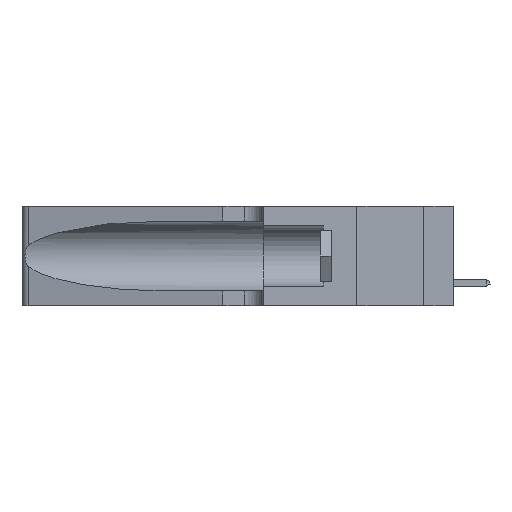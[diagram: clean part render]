
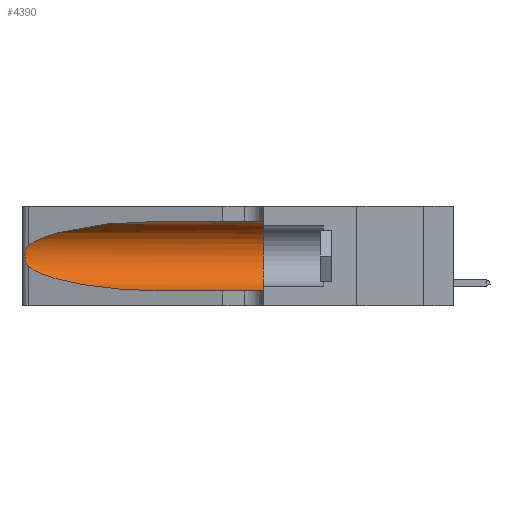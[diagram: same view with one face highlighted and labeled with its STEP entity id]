
A CAD part, left-side view. The second image highlights one B-rep face of the part: STEP entity #4390.
In plain terms, the highlighted cylindrical face has radius 3.308 mm (diameter 6.617 mm), a partial arc.
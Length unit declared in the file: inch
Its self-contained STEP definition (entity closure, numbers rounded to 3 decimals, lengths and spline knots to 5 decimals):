
#173 = CARTESIAN_POINT ( 'NONE',  ( 0.25487, 1.22718, 0.14631 ) ) ;
#246 = CARTESIAN_POINT ( 'NONE',  ( 0.26075, 1.23896, 0.178 ) ) ;
#338 = VERTEX_POINT ( 'NONE', #14343 ) ;
#577 = DIRECTION ( 'NONE',  ( 0., 0., 1. ) ) ;
#1189 = LINE ( 'NONE', #12483, #6958 ) ;
#2213 = CARTESIAN_POINT ( 'NONE',  ( 0.25487, 1.22718, 0.22369 ) ) ;
#2316 = AXIS2_PLACEMENT_3D ( 'NONE', #17102, #3715, #577 ) ;
#2671 = B_SPLINE_CURVE_WITH_KNOTS ( 'NONE', 3,
 ( #15286, #18796, #13555, #13475, #18503, #7005, #17047, #246, #20250, #18652, #7074, #10379, #8681, #8752 ),
 .UNSPECIFIED., .F., .F.,
 ( 4, 2, 2, 2, 2, 2, 4 ),
 ( 0., 0.00027, 0.00053, 0.00107, 0.0016, 0.00187, 0.00214 ),
 .UNSPECIFIED. ) ;
#3072 = CARTESIAN_POINT ( 'NONE',  ( 0.2373, 1.15595, 0.28018 ) ) ;
#3584 = CIRCLE ( 'NONE', #2316, 0.13025 ) ;
#3715 = DIRECTION ( 'NONE',  ( 0., 1., 0. ) ) ;
#4390 = ADVANCED_FACE ( 'NONE', ( #12271 ), #21081, .F. ) ;
#4749 = EDGE_CURVE ( 'NONE', #10232, #21205, #10947, .T. ) ;
#4982 = CARTESIAN_POINT ( 'NONE',  ( 0.1305, 0.35, 0.05475 ) ) ;
#5473 = VERTEX_POINT ( 'NONE', #2213 ) ;
#6452 = ORIENTED_EDGE ( 'NONE', *, *, #4749, .T. ) ;
#6772 = CARTESIAN_POINT ( 'NONE',  ( 0.1305, 1.61858, 0.185 ) ) ;
#6958 = VECTOR ( 'NONE', #9335, 39.37008 ) ;
#6992 = DIRECTION ( 'NONE',  ( 0., 0., -1. ) ) ;
#7005 = CARTESIAN_POINT ( 'NONE',  ( 0.26018, 1.23835, 0.19895 ) ) ;
#7065 = DIRECTION ( 'NONE',  ( 0., -1., 0. ) ) ;
#7074 = CARTESIAN_POINT ( 'NONE',  ( 0.25789, 1.23486, 0.15765 ) ) ;
#7789 = VECTOR ( 'NONE', #11862, 39.37008 ) ;
#7933 = CARTESIAN_POINT ( 'NONE',  ( 0.18966, 0.96281, 0.31525 ) ) ;
#8681 = CARTESIAN_POINT ( 'NONE',  ( 0.25555, 1.22993, 0.14849 ) ) ;
#8752 = CARTESIAN_POINT ( 'NONE',  ( 0.25487, 1.22718, 0.14631 ) ) ;
#9283 = ORIENTED_EDGE ( 'NONE', *, *, #18385, .F. ) ;
#9335 = DIRECTION ( 'NONE',  ( 0., -1., 0. ) ) ;
#9555 = CARTESIAN_POINT ( 'NONE',  ( 0.1305, 0.72297, 0.31525 ) ) ;
#10232 = VERTEX_POINT ( 'NONE', #15454 ) ;
#10379 = CARTESIAN_POINT ( 'NONE',  ( 0.25639, 1.23186, 0.15144 ) ) ;
#10515 = CARTESIAN_POINT ( 'NONE',  ( 0.1305, 0.72297, 0.31525 ) ) ;
#10947 = LINE ( 'NONE', #18692, #7789 ) ;
#11135 = ORIENTED_EDGE ( 'NONE', *, *, #15797, .T. ) ;
#11862 = DIRECTION ( 'NONE',  ( 0., -1., 0. ) ) ;
#12271 = FACE_OUTER_BOUND ( 'NONE', #17602, .T. ) ;
#12343 = ORIENTED_EDGE ( 'NONE', *, *, #18134, .F. ) ;
#12483 = CARTESIAN_POINT ( 'NONE',  ( 0.1305, 1.61858, 0.31525 ) ) ;
#13413 = ORIENTED_EDGE ( 'NONE', *, *, #18609, .T. ) ;
#13475 = CARTESIAN_POINT ( 'NONE',  ( 0.25787, 1.23484, 0.2124 ) ) ;
#13480 = CARTESIAN_POINT ( 'NONE',  ( 0.2373, 1.15595, 0.08982 ) ) ;
#13555 = CARTESIAN_POINT ( 'NONE',  ( 0.25639, 1.23184, 0.21858 ) ) ;
#14343 = CARTESIAN_POINT ( 'NONE',  ( 0.1305, 0.35, 0.31525 ) ) ;
#14991 = CARTESIAN_POINT ( 'NONE',  ( 0.25487, 1.22718, 0.22369 ) ) ;
#15113 = CARTESIAN_POINT ( 'NONE',  ( 0.25487, 1.22718, 0.14631 ) ) ;
#15213 =( BOUNDED_CURVE ( )  B_SPLINE_CURVE ( 3, ( #9555, #7933, #3072, #14991 ),
 .UNSPECIFIED., .F., .T. ) 
 B_SPLINE_CURVE_WITH_KNOTS ( ( 4, 4 ),
 ( 1.5708, 2.84003 ),
 .UNSPECIFIED. ) 
 CURVE ( )  GEOMETRIC_REPRESENTATION_ITEM ( )  RATIONAL_B_SPLINE_CURVE ( ( 1., 0.87, 0.87, 1. ) ) 
 REPRESENTATION_ITEM ( '' )  );
#15286 = CARTESIAN_POINT ( 'NONE',  ( 0.25487, 1.22718, 0.22369 ) ) ;
#15454 = CARTESIAN_POINT ( 'NONE',  ( 0.1305, 0.72297, 0.05475 ) ) ;
#15797 = EDGE_CURVE ( 'NONE', #5473, #18073, #2671, .T. ) ;
#16538 = CARTESIAN_POINT ( 'NONE',  ( 0.18966, 0.96281, 0.05475 ) ) ;
#16896 = AXIS2_PLACEMENT_3D ( 'NONE', #6772, #7065, #6992 ) ;
#17047 = CARTESIAN_POINT ( 'NONE',  ( 0.26075, 1.23896, 0.19203 ) ) ;
#17102 = CARTESIAN_POINT ( 'NONE',  ( 0.1305, 0.35, 0.185 ) ) ;
#17602 = EDGE_LOOP ( 'NONE', ( #18948, #11135, #13413, #6452, #12343, #9283 ) ) ;
#18073 = VERTEX_POINT ( 'NONE', #15113 ) ;
#18134 = EDGE_CURVE ( 'NONE', #338, #21205, #3584, .T. ) ;
#18385 = EDGE_CURVE ( 'NONE', #20696, #338, #1189, .T. ) ;
#18503 = CARTESIAN_POINT ( 'NONE',  ( 0.25854, 1.2359, 0.20912 ) ) ;
#18609 = EDGE_CURVE ( 'NONE', #18073, #10232, #20678, .T. ) ;
#18652 = CARTESIAN_POINT ( 'NONE',  ( 0.25856, 1.23593, 0.16098 ) ) ;
#18692 = CARTESIAN_POINT ( 'NONE',  ( 0.1305, 1.61858, 0.05475 ) ) ;
#18796 = CARTESIAN_POINT ( 'NONE',  ( 0.25555, 1.22994, 0.2215 ) ) ;
#18948 = ORIENTED_EDGE ( 'NONE', *, *, #20623, .T. ) ;
#19889 = CARTESIAN_POINT ( 'NONE',  ( 0.1305, 0.72297, 0.05475 ) ) ;
#20250 = CARTESIAN_POINT ( 'NONE',  ( 0.26017, 1.23833, 0.17102 ) ) ;
#20623 = EDGE_CURVE ( 'NONE', #20696, #5473, #15213, .T. ) ;
#20678 =( BOUNDED_CURVE ( )  B_SPLINE_CURVE ( 3, ( #173, #13480, #16538, #19889 ),
 .UNSPECIFIED., .F., .T. ) 
 B_SPLINE_CURVE_WITH_KNOTS ( ( 4, 4 ),
 ( 3.44316, 4.71239 ),
 .UNSPECIFIED. ) 
 CURVE ( )  GEOMETRIC_REPRESENTATION_ITEM ( )  RATIONAL_B_SPLINE_CURVE ( ( 1., 0.87, 0.87, 1. ) ) 
 REPRESENTATION_ITEM ( '' )  );
#20696 = VERTEX_POINT ( 'NONE', #10515 ) ;
#21081 = CYLINDRICAL_SURFACE ( 'NONE', #16896, 0.13025 ) ;
#21205 = VERTEX_POINT ( 'NONE', #4982 ) ;
